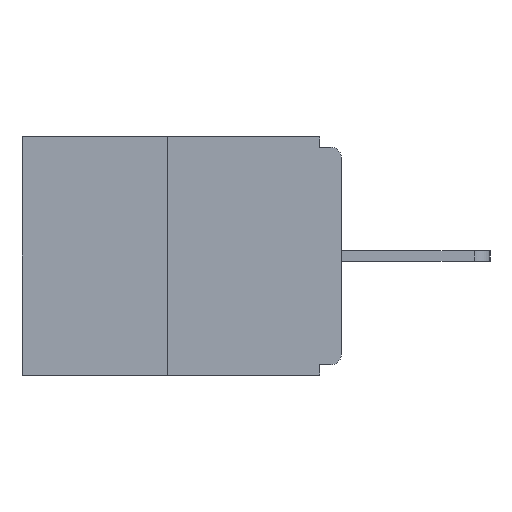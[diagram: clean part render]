
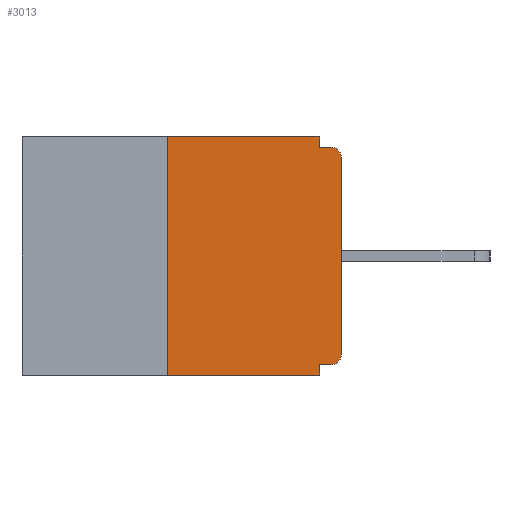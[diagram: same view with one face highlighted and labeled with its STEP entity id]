
A CAD part, left-side view. The second image highlights one B-rep face of the part: STEP entity #3013.
In plain terms, the highlighted planar face has unit normal (-1, 0, 0).
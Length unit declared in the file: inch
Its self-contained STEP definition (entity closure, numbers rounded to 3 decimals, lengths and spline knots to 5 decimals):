
#65 = VECTOR ( 'NONE', #18228, 39.37008 ) ;
#531 = VECTOR ( 'NONE', #9957, 39.37008 ) ;
#673 = CARTESIAN_POINT ( 'NONE',  ( 0., 0.031, -0.015 ) ) ;
#792 = CARTESIAN_POINT ( 'NONE',  ( 0., 0.031, 0. ) ) ;
#844 = PLANE ( 'NONE',  #11635 ) ;
#924 = AXIS2_PLACEMENT_3D ( 'NONE', #19983, #26183, #26320 ) ;
#1674 = CARTESIAN_POINT ( 'NONE',  ( 0., 0.46, 0. ) ) ;
#2089 = LINE ( 'NONE', #10711, #10270 ) ;
#2852 = FACE_OUTER_BOUND ( 'NONE', #2922, .T. ) ;
#2922 = EDGE_LOOP ( 'NONE', ( #21698, #23268, #17222, #9939, #9507, #26118, #12206, #22744, #12572, #24850 ) ) ;
#3008 = CARTESIAN_POINT ( 'NONE',  ( 0., 0., -0.313 ) ) ;
#3013 = ADVANCED_FACE ( 'NONE', ( #2852 ), #844, .F. ) ;
#3525 = AXIS2_PLACEMENT_3D ( 'NONE', #11941, #18418, #6630 ) ;
#3845 = CARTESIAN_POINT ( 'NONE',  ( 0., 0.031, -0.343 ) ) ;
#3986 = EDGE_CURVE ( 'NONE', #7476, #12987, #14365, .T. ) ;
#4507 = CARTESIAN_POINT ( 'NONE',  ( 0., 0.25, 0. ) ) ;
#4970 = DIRECTION ( 'NONE',  ( 0., 1., 0. ) ) ;
#5237 = LINE ( 'NONE', #7403, #7588 ) ;
#5284 = DIRECTION ( 'NONE',  ( 0., 0., -1. ) ) ;
#5876 = DIRECTION ( 'NONE',  ( 0., -1., 0. ) ) ;
#6026 = CARTESIAN_POINT ( 'NONE',  ( 0., 0.015, -0.015 ) ) ;
#6433 = CARTESIAN_POINT ( 'NONE',  ( 0., 0.25, 0. ) ) ;
#6502 = VECTOR ( 'NONE', #18544, 39.37008 ) ;
#6531 = CARTESIAN_POINT ( 'NONE',  ( 0., 0.031, 0. ) ) ;
#6630 = DIRECTION ( 'NONE',  ( 0., 0., -1. ) ) ;
#7403 = CARTESIAN_POINT ( 'NONE',  ( 0., 0., -0.328 ) ) ;
#7476 = VERTEX_POINT ( 'NONE', #4507 ) ;
#7588 = VECTOR ( 'NONE', #4970, 39.37008 ) ;
#7685 = CARTESIAN_POINT ( 'NONE',  ( 0., 0.015, -0.328 ) ) ;
#9099 = CIRCLE ( 'NONE', #924, 0.015 ) ;
#9507 = ORIENTED_EDGE ( 'NONE', *, *, #25030, .F. ) ;
#9899 = EDGE_CURVE ( 'NONE', #17556, #20715, #20344, .T. ) ;
#9939 = ORIENTED_EDGE ( 'NONE', *, *, #11719, .F. ) ;
#9957 = DIRECTION ( 'NONE',  ( 0., 0., -1. ) ) ;
#10270 = VECTOR ( 'NONE', #20972, 39.37008 ) ;
#10711 = CARTESIAN_POINT ( 'NONE',  ( 0., 0.031, -0.343 ) ) ;
#10998 = VERTEX_POINT ( 'NONE', #15095 ) ;
#11529 = VECTOR ( 'NONE', #12781, 39.37008 ) ;
#11635 = AXIS2_PLACEMENT_3D ( 'NONE', #15293, #19734, #5284 ) ;
#11719 = EDGE_CURVE ( 'NONE', #20835, #12931, #2089, .T. ) ;
#11941 = CARTESIAN_POINT ( 'NONE',  ( 0., 0.015, -0.03 ) ) ;
#12182 = VECTOR ( 'NONE', #21855, 39.37008 ) ;
#12206 = ORIENTED_EDGE ( 'NONE', *, *, #17697, .T. ) ;
#12572 = ORIENTED_EDGE ( 'NONE', *, *, #9899, .F. ) ;
#12595 = EDGE_CURVE ( 'NONE', #10998, #7476, #20880, .T. ) ;
#12781 = DIRECTION ( 'NONE',  ( 0., 0., 1. ) ) ;
#12931 = VERTEX_POINT ( 'NONE', #3845 ) ;
#12987 = VERTEX_POINT ( 'NONE', #6531 ) ;
#13621 = LINE ( 'NONE', #16076, #12182 ) ;
#13916 = VECTOR ( 'NONE', #5876, 39.37008 ) ;
#14365 = LINE ( 'NONE', #1674, #6502 ) ;
#15095 = CARTESIAN_POINT ( 'NONE',  ( 0., 0.25, -0.343 ) ) ;
#15293 = CARTESIAN_POINT ( 'NONE',  ( 0., 0.46, 0. ) ) ;
#16076 = CARTESIAN_POINT ( 'NONE',  ( 0., 0., 0. ) ) ;
#16344 = CARTESIAN_POINT ( 'NONE',  ( 0., 0.46, -0.343 ) ) ;
#16480 = LINE ( 'NONE', #16344, #65 ) ;
#16843 = EDGE_CURVE ( 'NONE', #16885, #23014, #9099, .T. ) ;
#16874 = EDGE_CURVE ( 'NONE', #10998, #12931, #16480, .T. ) ;
#16885 = VERTEX_POINT ( 'NONE', #7685 ) ;
#17222 = ORIENTED_EDGE ( 'NONE', *, *, #16874, .T. ) ;
#17556 = VERTEX_POINT ( 'NONE', #673 ) ;
#17689 = CARTESIAN_POINT ( 'NONE',  ( 0., 0., -0.03 ) ) ;
#17697 = EDGE_CURVE ( 'NONE', #23014, #18781, #13621, .T. ) ;
#18228 = DIRECTION ( 'NONE',  ( 0., -1., 0. ) ) ;
#18418 = DIRECTION ( 'NONE',  ( -1., 0., 0. ) ) ;
#18544 = DIRECTION ( 'NONE',  ( 0., -1., 0. ) ) ;
#18604 = EDGE_CURVE ( 'NONE', #18781, #20715, #22943, .T. ) ;
#18781 = VERTEX_POINT ( 'NONE', #17689 ) ;
#19269 = EDGE_CURVE ( 'NONE', #12987, #17556, #19285, .T. ) ;
#19285 = LINE ( 'NONE', #792, #531 ) ;
#19734 = DIRECTION ( 'NONE',  ( 1., 0., 0. ) ) ;
#19983 = CARTESIAN_POINT ( 'NONE',  ( 0., 0.015, -0.313 ) ) ;
#20344 = LINE ( 'NONE', #24395, #13916 ) ;
#20715 = VERTEX_POINT ( 'NONE', #6026 ) ;
#20835 = VERTEX_POINT ( 'NONE', #25327 ) ;
#20880 = LINE ( 'NONE', #6433, #11529 ) ;
#20972 = DIRECTION ( 'NONE',  ( 0., 0., -1. ) ) ;
#21698 = ORIENTED_EDGE ( 'NONE', *, *, #3986, .F. ) ;
#21855 = DIRECTION ( 'NONE',  ( 0., 0., 1. ) ) ;
#22744 = ORIENTED_EDGE ( 'NONE', *, *, #18604, .T. ) ;
#22943 = CIRCLE ( 'NONE', #3525, 0.015 ) ;
#23014 = VERTEX_POINT ( 'NONE', #3008 ) ;
#23268 = ORIENTED_EDGE ( 'NONE', *, *, #12595, .F. ) ;
#24395 = CARTESIAN_POINT ( 'NONE',  ( 0., 0., -0.015 ) ) ;
#24850 = ORIENTED_EDGE ( 'NONE', *, *, #19269, .F. ) ;
#25030 = EDGE_CURVE ( 'NONE', #16885, #20835, #5237, .T. ) ;
#25327 = CARTESIAN_POINT ( 'NONE',  ( 0., 0.031, -0.328 ) ) ;
#26118 = ORIENTED_EDGE ( 'NONE', *, *, #16843, .T. ) ;
#26183 = DIRECTION ( 'NONE',  ( -1., 0., 0. ) ) ;
#26320 = DIRECTION ( 'NONE',  ( 0., 0., -1. ) ) ;
